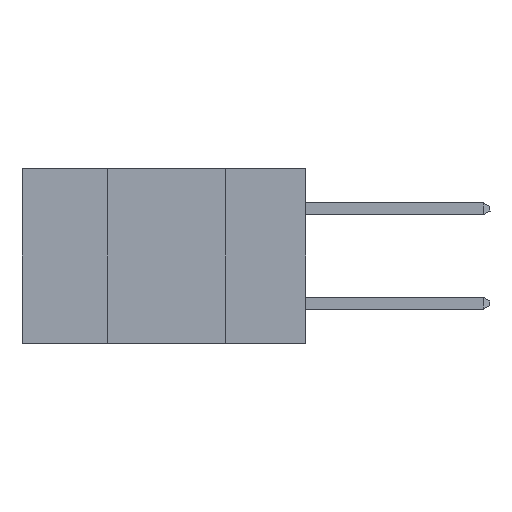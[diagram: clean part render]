
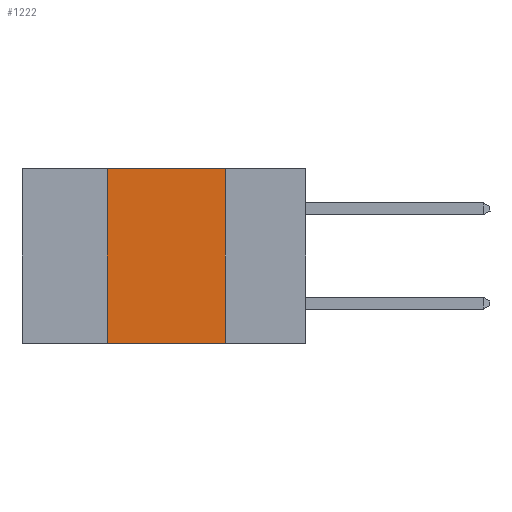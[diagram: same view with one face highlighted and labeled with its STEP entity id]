
A CAD part, left-side view. The second image highlights one B-rep face of the part: STEP entity #1222.
In plain terms, the highlighted planar face has unit normal (-1, 0, 0).
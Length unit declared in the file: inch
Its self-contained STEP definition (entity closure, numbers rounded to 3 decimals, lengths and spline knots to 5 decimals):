
#124 = CARTESIAN_POINT ( 'NONE',  ( 0., 0.42, 0. ) ) ;
#1222 = ADVANCED_FACE ( 'NONE', ( #11603 ), #15121, .F. ) ;
#1706 = DIRECTION ( 'NONE',  ( 0., -1., 0. ) ) ;
#3036 = CARTESIAN_POINT ( 'NONE',  ( 0., 0.17, -0.37 ) ) ;
#3242 = ORIENTED_EDGE ( 'NONE', *, *, #3555, .F. ) ;
#3555 = EDGE_CURVE ( 'NONE', #8470, #13274, #10995, .T. ) ;
#3585 = VECTOR ( 'NONE', #11069, 39.37008 ) ;
#4421 = EDGE_CURVE ( 'NONE', #11761, #6409, #17372, .T. ) ;
#4730 = CARTESIAN_POINT ( 'NONE',  ( 0., 0.42, -0.37 ) ) ;
#5800 = CARTESIAN_POINT ( 'NONE',  ( 0., 0.6, -0.37 ) ) ;
#6174 = EDGE_LOOP ( 'NONE', ( #3242, #10810, #9817, #7588 ) ) ;
#6409 = VERTEX_POINT ( 'NONE', #12730 ) ;
#6884 = VECTOR ( 'NONE', #1706, 39.37008 ) ;
#6907 = CARTESIAN_POINT ( 'NONE',  ( 0., 0.6, 0. ) ) ;
#7588 = ORIENTED_EDGE ( 'NONE', *, *, #14696, .T. ) ;
#8338 = DIRECTION ( 'NONE',  ( 1., 0., 0. ) ) ;
#8470 = VERTEX_POINT ( 'NONE', #16152 ) ;
#8596 = DIRECTION ( 'NONE',  ( 0., 0., -1. ) ) ;
#9817 = ORIENTED_EDGE ( 'NONE', *, *, #4421, .F. ) ;
#10810 = ORIENTED_EDGE ( 'NONE', *, *, #17468, .F. ) ;
#10960 = LINE ( 'NONE', #5800, #6884 ) ;
#10995 = LINE ( 'NONE', #12632, #12720 ) ;
#11069 = DIRECTION ( 'NONE',  ( 0., -1., 0. ) ) ;
#11603 = FACE_OUTER_BOUND ( 'NONE', #6174, .T. ) ;
#11761 = VERTEX_POINT ( 'NONE', #4730 ) ;
#12511 = CARTESIAN_POINT ( 'NONE',  ( 0., 0.6, 0. ) ) ;
#12632 = CARTESIAN_POINT ( 'NONE',  ( 0., 0.17, 0. ) ) ;
#12720 = VECTOR ( 'NONE', #8596, 39.37008 ) ;
#12730 = CARTESIAN_POINT ( 'NONE',  ( 0., 0.42, 0. ) ) ;
#13274 = VERTEX_POINT ( 'NONE', #3036 ) ;
#13827 = DIRECTION ( 'NONE',  ( 0., 0., 1. ) ) ;
#13883 = LINE ( 'NONE', #12511, #3585 ) ;
#14696 = EDGE_CURVE ( 'NONE', #11761, #13274, #10960, .T. ) ;
#15121 = PLANE ( 'NONE',  #15954 ) ;
#15954 = AXIS2_PLACEMENT_3D ( 'NONE', #6907, #8338, #16503 ) ;
#16152 = CARTESIAN_POINT ( 'NONE',  ( 0., 0.17, 0. ) ) ;
#16503 = DIRECTION ( 'NONE',  ( 0., 0., -1. ) ) ;
#16538 = VECTOR ( 'NONE', #13827, 39.37008 ) ;
#17372 = LINE ( 'NONE', #124, #16538 ) ;
#17468 = EDGE_CURVE ( 'NONE', #6409, #8470, #13883, .T. ) ;
